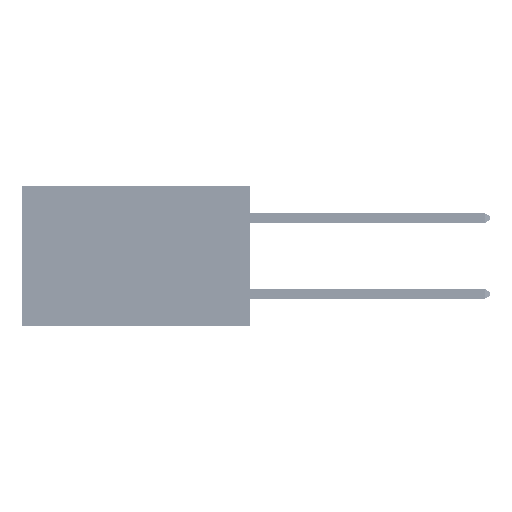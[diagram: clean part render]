
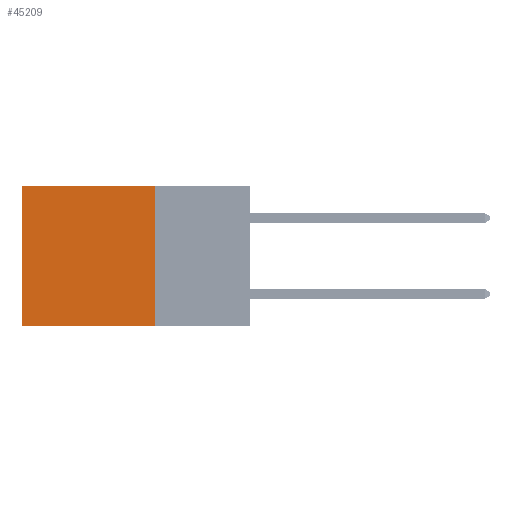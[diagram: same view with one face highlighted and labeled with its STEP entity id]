
A CAD part, left-side view. The second image highlights one B-rep face of the part: STEP entity #45209.
In plain terms, the highlighted planar face has unit normal (-1, 0, 0).
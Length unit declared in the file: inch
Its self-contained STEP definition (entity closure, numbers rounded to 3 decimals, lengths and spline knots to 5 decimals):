
#440 = ORIENTED_EDGE ( 'NONE', *, *, #12037, .F. ) ;
#489 = VERTEX_POINT ( 'NONE', #29377 ) ;
#732 = EDGE_CURVE ( 'NONE', #28600, #3917, #3883, .T. ) ;
#1221 = DIRECTION ( 'NONE',  ( 0., 0., -1. ) ) ;
#1631 = CARTESIAN_POINT ( 'NONE',  ( 0.2875, 0.25, -0.37 ) ) ;
#3883 = LINE ( 'NONE', #22565, #44912 ) ;
#3917 = VERTEX_POINT ( 'NONE', #6587 ) ;
#6376 = DIRECTION ( 'NONE',  ( 0., 0., -1. ) ) ;
#6587 = CARTESIAN_POINT ( 'NONE',  ( 0.2875, 0.6, 0. ) ) ;
#7930 = EDGE_LOOP ( 'NONE', ( #49380, #440, #21649, #16699 ) ) ;
#9547 = CARTESIAN_POINT ( 'NONE',  ( 0.2875, 0.6, 0. ) ) ;
#9560 = VECTOR ( 'NONE', #22231, 39.37008 ) ;
#10434 = EDGE_CURVE ( 'NONE', #28600, #50188, #50915, .T. ) ;
#12037 = EDGE_CURVE ( 'NONE', #50188, #489, #20534, .T. ) ;
#12559 = CARTESIAN_POINT ( 'NONE',  ( 0.2875, 0.25, 0. ) ) ;
#16699 = ORIENTED_EDGE ( 'NONE', *, *, #732, .T. ) ;
#20534 = LINE ( 'NONE', #1631, #9560 ) ;
#20845 = VECTOR ( 'NONE', #1221, 39.37008 ) ;
#21649 = ORIENTED_EDGE ( 'NONE', *, *, #10434, .F. ) ;
#22231 = DIRECTION ( 'NONE',  ( 0., 1., 0. ) ) ;
#22565 = CARTESIAN_POINT ( 'NONE',  ( 0.2875, 0.25, 0. ) ) ;
#22791 = PLANE ( 'NONE',  #23661 ) ;
#23661 = AXIS2_PLACEMENT_3D ( 'NONE', #51280, #30985, #6376 ) ;
#24995 = DIRECTION ( 'NONE',  ( 0., 0., -1. ) ) ;
#28600 = VERTEX_POINT ( 'NONE', #12559 ) ;
#29377 = CARTESIAN_POINT ( 'NONE',  ( 0.2875, 0.6, -0.37 ) ) ;
#30985 = DIRECTION ( 'NONE',  ( 1., 0., 0. ) ) ;
#35027 = CARTESIAN_POINT ( 'NONE',  ( 0.2875, 0.25, -0.37 ) ) ;
#35582 = LINE ( 'NONE', #9547, #20845 ) ;
#38850 = VECTOR ( 'NONE', #24995, 39.37008 ) ;
#42794 = FACE_OUTER_BOUND ( 'NONE', #7930, .T. ) ;
#44912 = VECTOR ( 'NONE', #46978, 39.37008 ) ;
#45209 = ADVANCED_FACE ( 'NONE', ( #42794 ), #22791, .F. ) ;
#45277 = CARTESIAN_POINT ( 'NONE',  ( 0.2875, 0.25, 0. ) ) ;
#46978 = DIRECTION ( 'NONE',  ( 0., 1., 0. ) ) ;
#48084 = EDGE_CURVE ( 'NONE', #3917, #489, #35582, .T. ) ;
#49380 = ORIENTED_EDGE ( 'NONE', *, *, #48084, .T. ) ;
#50188 = VERTEX_POINT ( 'NONE', #35027 ) ;
#50915 = LINE ( 'NONE', #45277, #38850 ) ;
#51280 = CARTESIAN_POINT ( 'NONE',  ( 0.2875, 0.25, 0. ) ) ;
